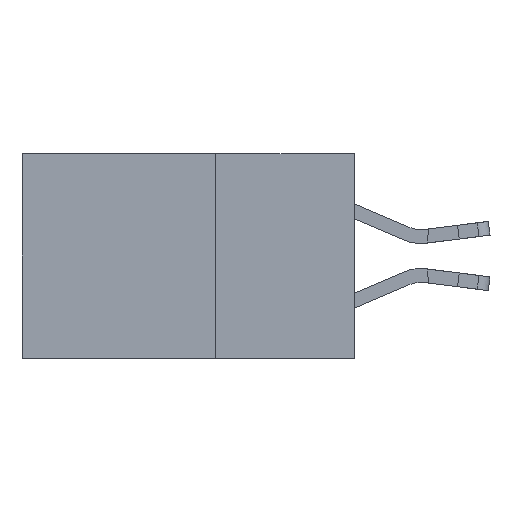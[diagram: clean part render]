
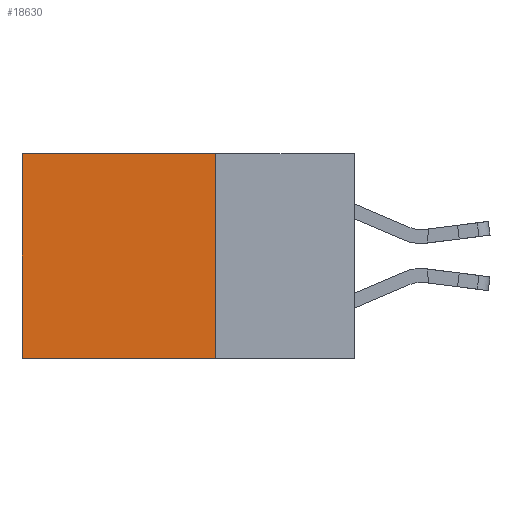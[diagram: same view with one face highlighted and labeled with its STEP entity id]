
A CAD part, left-side view. The second image highlights one B-rep face of the part: STEP entity #18630.
In plain terms, the highlighted planar face has unit normal (-1, 0, 0).
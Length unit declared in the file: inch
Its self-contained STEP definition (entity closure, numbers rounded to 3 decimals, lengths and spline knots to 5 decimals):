
#1168 = CARTESIAN_POINT ( 'NONE',  ( 0.298, 0.6, -0.37 ) ) ;
#1485 = DIRECTION ( 'NONE',  ( 0., 0., -1. ) ) ;
#1526 = EDGE_CURVE ( 'NONE', #19237, #3725, #5677, .T. ) ;
#1620 = FACE_OUTER_BOUND ( 'NONE', #6210, .T. ) ;
#3041 = CARTESIAN_POINT ( 'NONE',  ( 0.298, 0.25, -0.37 ) ) ;
#3437 = AXIS2_PLACEMENT_3D ( 'NONE', #13408, #26049, #13587 ) ;
#3718 = VECTOR ( 'NONE', #24021, 39.37008 ) ;
#3725 = VERTEX_POINT ( 'NONE', #12368 ) ;
#5630 = CARTESIAN_POINT ( 'NONE',  ( 0.298, 0.6, 0. ) ) ;
#5677 = LINE ( 'NONE', #21059, #16837 ) ;
#6210 = EDGE_LOOP ( 'NONE', ( #18821, #25556, #18904, #16960 ) ) ;
#9497 = VERTEX_POINT ( 'NONE', #18572 ) ;
#9983 = LINE ( 'NONE', #3041, #3718 ) ;
#11086 = VERTEX_POINT ( 'NONE', #1168 ) ;
#11227 = LINE ( 'NONE', #5630, #21045 ) ;
#12368 = CARTESIAN_POINT ( 'NONE',  ( 0.298, 0.25, -0.37 ) ) ;
#12640 = EDGE_CURVE ( 'NONE', #19237, #9497, #23366, .T. ) ;
#13280 = CARTESIAN_POINT ( 'NONE',  ( 0.298, 0.25, 0. ) ) ;
#13408 = CARTESIAN_POINT ( 'NONE',  ( 0.298, 0.25, 0. ) ) ;
#13587 = DIRECTION ( 'NONE',  ( 0., 0., -1. ) ) ;
#16324 = EDGE_CURVE ( 'NONE', #3725, #11086, #9983, .T. ) ;
#16719 = DIRECTION ( 'NONE',  ( 0., 1., 0. ) ) ;
#16837 = VECTOR ( 'NONE', #21002, 39.37008 ) ;
#16960 = ORIENTED_EDGE ( 'NONE', *, *, #12640, .T. ) ;
#17854 = VECTOR ( 'NONE', #16719, 39.37008 ) ;
#18572 = CARTESIAN_POINT ( 'NONE',  ( 0.298, 0.6, 0. ) ) ;
#18630 = ADVANCED_FACE ( 'NONE', ( #1620 ), #23984, .F. ) ;
#18809 = CARTESIAN_POINT ( 'NONE',  ( 0.298, 0.25, 0. ) ) ;
#18821 = ORIENTED_EDGE ( 'NONE', *, *, #23634, .T. ) ;
#18904 = ORIENTED_EDGE ( 'NONE', *, *, #1526, .F. ) ;
#19237 = VERTEX_POINT ( 'NONE', #13280 ) ;
#21002 = DIRECTION ( 'NONE',  ( 0., 0., -1. ) ) ;
#21045 = VECTOR ( 'NONE', #1485, 39.37008 ) ;
#21059 = CARTESIAN_POINT ( 'NONE',  ( 0.298, 0.25, 0. ) ) ;
#23366 = LINE ( 'NONE', #18809, #17854 ) ;
#23634 = EDGE_CURVE ( 'NONE', #9497, #11086, #11227, .T. ) ;
#23984 = PLANE ( 'NONE',  #3437 ) ;
#24021 = DIRECTION ( 'NONE',  ( 0., 1., 0. ) ) ;
#25556 = ORIENTED_EDGE ( 'NONE', *, *, #16324, .F. ) ;
#26049 = DIRECTION ( 'NONE',  ( 1., 0., 0. ) ) ;
